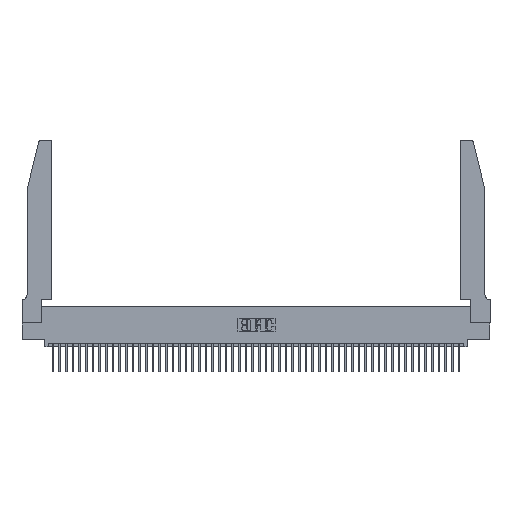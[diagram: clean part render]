
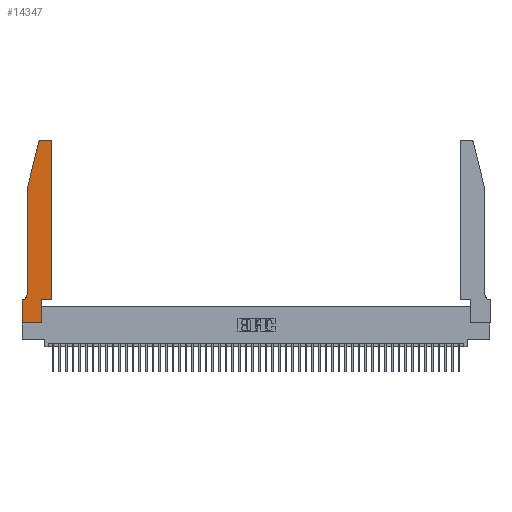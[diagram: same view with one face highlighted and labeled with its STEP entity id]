
A CAD part, top view. The second image highlights one B-rep face of the part: STEP entity #14347.
In plain terms, the highlighted planar face has unit normal (0, 0, 1).
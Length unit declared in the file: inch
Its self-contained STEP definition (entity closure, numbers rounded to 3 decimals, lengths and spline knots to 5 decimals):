
#776 = DIRECTION ( 'NONE',  ( -1., 0., 0. ) ) ;
#1335 = FACE_OUTER_BOUND ( 'NONE', #7827, .T. ) ;
#1978 = CIRCLE ( 'NONE', #24730, 0.03 ) ;
#2772 = VERTEX_POINT ( 'NONE', #25679 ) ;
#4658 = VERTEX_POINT ( 'NONE', #36267 ) ;
#5137 = EDGE_CURVE ( 'NONE', #4658, #12374, #17161, .T. ) ;
#5824 = VECTOR ( 'NONE', #31085, 39.37008 ) ;
#6303 = VERTEX_POINT ( 'NONE', #12582 ) ;
#7827 = EDGE_LOOP ( 'NONE', ( #44224, #50231, #42745, #23714, #26040, #29005, #46735, #19988, #14542, #36626, #28965, #11294 ) ) ;
#8557 = DIRECTION ( 'NONE',  ( 0., -1., 0. ) ) ;
#8666 = LINE ( 'NONE', #33947, #30749 ) ;
#8911 = EDGE_CURVE ( 'NONE', #2772, #32194, #48683, .T. ) ;
#9394 = CARTESIAN_POINT ( 'NONE',  ( 0.2865, 0., 0.37 ) ) ;
#11028 = VECTOR ( 'NONE', #37190, 39.37008 ) ;
#11294 = ORIENTED_EDGE ( 'NONE', *, *, #19879, .T. ) ;
#11650 = DIRECTION ( 'NONE',  ( -1., 0., 0. ) ) ;
#11831 = CARTESIAN_POINT ( 'NONE',  ( 0.0755, 2., 0.37 ) ) ;
#12374 = VERTEX_POINT ( 'NONE', #35192 ) ;
#12582 = CARTESIAN_POINT ( 'NONE',  ( 0.0755, 2., 0.37 ) ) ;
#12645 = DIRECTION ( 'NONE',  ( 0., 0., 1. ) ) ;
#12665 = VECTOR ( 'NONE', #32491, 39.37008 ) ;
#12838 = EDGE_CURVE ( 'NONE', #23635, #2772, #28494, .T. ) ;
#14347 = ADVANCED_FACE ( 'NONE', ( #1335 ), #47840, .T. ) ;
#14542 = ORIENTED_EDGE ( 'NONE', *, *, #28546, .T. ) ;
#14549 = CARTESIAN_POINT ( 'NONE',  ( 0.284, 2.72, 0.37 ) ) ;
#14604 = VERTEX_POINT ( 'NONE', #45442 ) ;
#15224 = CARTESIAN_POINT ( 'NONE',  ( 0.4505, 0.35, 0.37 ) ) ;
#15536 = CARTESIAN_POINT ( 'NONE',  ( 0.4505, 2.72, 0.37 ) ) ;
#17161 = LINE ( 'NONE', #41153, #11028 ) ;
#19410 = DIRECTION ( 'NONE',  ( -1., 0., 0. ) ) ;
#19879 = EDGE_CURVE ( 'NONE', #22736, #23635, #1978, .T. ) ;
#19988 = ORIENTED_EDGE ( 'NONE', *, *, #31729, .T. ) ;
#20300 = VERTEX_POINT ( 'NONE', #30151 ) ;
#22376 = DIRECTION ( 'NONE',  ( 0., 1., 0. ) ) ;
#22736 = VERTEX_POINT ( 'NONE', #15536 ) ;
#23022 = CARTESIAN_POINT ( 'NONE',  ( 0.2605, 2.75, 0.37 ) ) ;
#23277 = AXIS2_PLACEMENT_3D ( 'NONE', #36166, #12645, #48177 ) ;
#23337 = CARTESIAN_POINT ( 'NONE',  ( 0.0755, 2., 0.37 ) ) ;
#23523 = LINE ( 'NONE', #36358, #35821 ) ;
#23634 = CARTESIAN_POINT ( 'NONE',  ( 0.4205, 2.72, 0.37 ) ) ;
#23635 = VERTEX_POINT ( 'NONE', #28365 ) ;
#23714 = ORIENTED_EDGE ( 'NONE', *, *, #27329, .T. ) ;
#24730 = AXIS2_PLACEMENT_3D ( 'NONE', #23634, #27580, #27751 ) ;
#25679 = CARTESIAN_POINT ( 'NONE',  ( 0.284, 2.75, 0.37 ) ) ;
#25924 = EDGE_CURVE ( 'NONE', #12374, #22736, #47745, .T. ) ;
#26040 = ORIENTED_EDGE ( 'NONE', *, *, #42128, .T. ) ;
#26394 = CIRCLE ( 'NONE', #36248, 0.07 ) ;
#26920 = DIRECTION ( 'NONE',  ( 0., 0., -1. ) ) ;
#27230 = CARTESIAN_POINT ( 'NONE',  ( 0.25487, 2.72718, 0.37 ) ) ;
#27329 = EDGE_CURVE ( 'NONE', #6303, #14604, #34721, .T. ) ;
#27580 = DIRECTION ( 'NONE',  ( 0., 0., 1. ) ) ;
#27751 = DIRECTION ( 'NONE',  ( 1., 0., 0. ) ) ;
#28144 = VECTOR ( 'NONE', #39635, 39.37008 ) ;
#28365 = CARTESIAN_POINT ( 'NONE',  ( 0.4205, 2.75, 0.37 ) ) ;
#28494 = LINE ( 'NONE', #23022, #38409 ) ;
#28546 = EDGE_CURVE ( 'NONE', #47020, #4658, #8666, .T. ) ;
#28808 = CARTESIAN_POINT ( 'NONE',  ( 0., 0., 0.37 ) ) ;
#28965 = ORIENTED_EDGE ( 'NONE', *, *, #25924, .T. ) ;
#29005 = ORIENTED_EDGE ( 'NONE', *, *, #45804, .T. ) ;
#29286 = LINE ( 'NONE', #44490, #12665 ) ;
#30020 = DIRECTION ( 'NONE',  ( 1., 0., 0. ) ) ;
#30143 = EDGE_CURVE ( 'NONE', #32194, #6303, #44808, .T. ) ;
#30151 = CARTESIAN_POINT ( 'NONE',  ( 0., 0., 0.37 ) ) ;
#30286 = EDGE_CURVE ( 'NONE', #35376, #20300, #42336, .T. ) ;
#30347 = DIRECTION ( 'NONE',  ( 0., 0., 1. ) ) ;
#30749 = VECTOR ( 'NONE', #22376, 39.37008 ) ;
#31085 = DIRECTION ( 'NONE',  ( 0., -1., 0. ) ) ;
#31729 = EDGE_CURVE ( 'NONE', #20300, #47020, #29286, .T. ) ;
#32194 = VERTEX_POINT ( 'NONE', #27230 ) ;
#32491 = DIRECTION ( 'NONE',  ( 1., 0., 0. ) ) ;
#33947 = CARTESIAN_POINT ( 'NONE',  ( 0.2865, 0.35, 0.37 ) ) ;
#34721 = LINE ( 'NONE', #23337, #5824 ) ;
#35192 = CARTESIAN_POINT ( 'NONE',  ( 0.4505, 0.35, 0.37 ) ) ;
#35376 = VERTEX_POINT ( 'NONE', #39588 ) ;
#35550 = VECTOR ( 'NONE', #8557, 39.37008 ) ;
#35608 = AXIS2_PLACEMENT_3D ( 'NONE', #14549, #30347, #30020 ) ;
#35821 = VECTOR ( 'NONE', #776, 39.37008 ) ;
#36166 = CARTESIAN_POINT ( 'NONE',  ( 0., 0.35, 0.37 ) ) ;
#36248 = AXIS2_PLACEMENT_3D ( 'NONE', #43237, #26920, #11650 ) ;
#36267 = CARTESIAN_POINT ( 'NONE',  ( 0.2865, 0.35, 0.37 ) ) ;
#36358 = CARTESIAN_POINT ( 'NONE',  ( 0.0755, 0.35, 0.37 ) ) ;
#36626 = ORIENTED_EDGE ( 'NONE', *, *, #5137, .T. ) ;
#37190 = DIRECTION ( 'NONE',  ( 1., 0., 0. ) ) ;
#38162 = VERTEX_POINT ( 'NONE', #45342 ) ;
#38409 = VECTOR ( 'NONE', #19410, 39.37008 ) ;
#39588 = CARTESIAN_POINT ( 'NONE',  ( 0., 0.35, 0.37 ) ) ;
#39635 = DIRECTION ( 'NONE',  ( -0.239, -0.971, 0. ) ) ;
#41153 = CARTESIAN_POINT ( 'NONE',  ( 0.4505, 0.35, 0.37 ) ) ;
#41556 = DIRECTION ( 'NONE',  ( 0., 1., 0. ) ) ;
#42128 = EDGE_CURVE ( 'NONE', #14604, #38162, #26394, .T. ) ;
#42336 = LINE ( 'NONE', #28808, #35550 ) ;
#42745 = ORIENTED_EDGE ( 'NONE', *, *, #30143, .T. ) ;
#43237 = CARTESIAN_POINT ( 'NONE',  ( 0.0055, 0.42, 0.37 ) ) ;
#44224 = ORIENTED_EDGE ( 'NONE', *, *, #12838, .T. ) ;
#44490 = CARTESIAN_POINT ( 'NONE',  ( 0., 0., 0.37 ) ) ;
#44808 = LINE ( 'NONE', #11831, #28144 ) ;
#45342 = CARTESIAN_POINT ( 'NONE',  ( 0.0055, 0.35, 0.37 ) ) ;
#45442 = CARTESIAN_POINT ( 'NONE',  ( 0.0755, 0.42, 0.37 ) ) ;
#45804 = EDGE_CURVE ( 'NONE', #38162, #35376, #23523, .T. ) ;
#46512 = VECTOR ( 'NONE', #41556, 39.37008 ) ;
#46735 = ORIENTED_EDGE ( 'NONE', *, *, #30286, .T. ) ;
#47020 = VERTEX_POINT ( 'NONE', #9394 ) ;
#47745 = LINE ( 'NONE', #15224, #46512 ) ;
#47840 = PLANE ( 'NONE',  #23277 ) ;
#48177 = DIRECTION ( 'NONE',  ( 1., 0., 0. ) ) ;
#48683 = CIRCLE ( 'NONE', #35608, 0.03 ) ;
#50231 = ORIENTED_EDGE ( 'NONE', *, *, #8911, .T. ) ;
